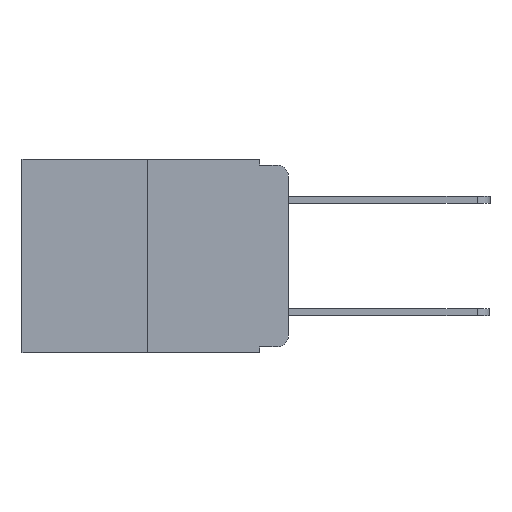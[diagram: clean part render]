
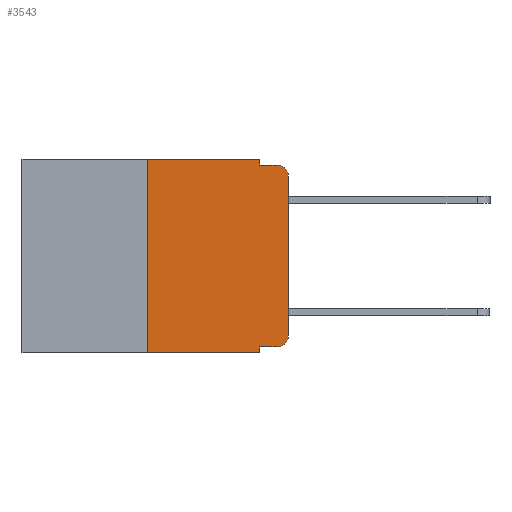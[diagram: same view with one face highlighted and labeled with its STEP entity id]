
A CAD part, left-side view. The second image highlights one B-rep face of the part: STEP entity #3543.
In plain terms, the highlighted planar face has unit normal (-1, 0, 0).
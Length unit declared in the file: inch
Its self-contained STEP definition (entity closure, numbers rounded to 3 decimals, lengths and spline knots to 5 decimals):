
#11 = VECTOR ( 'NONE', #3210, 39.37008 ) ;
#379 = VERTEX_POINT ( 'NONE', #9284 ) ;
#390 = DIRECTION ( 'NONE',  ( 0., -1., 0. ) ) ;
#411 = VERTEX_POINT ( 'NONE', #7543 ) ;
#413 = VECTOR ( 'NONE', #2440, 39.37008 ) ;
#439 = CIRCLE ( 'NONE', #7795, 0.02 ) ;
#510 = CARTESIAN_POINT ( 'NONE',  ( 0., 0.25, -0.343 ) ) ;
#577 = EDGE_CURVE ( 'NONE', #2965, #7936, #9200, .T. ) ;
#723 = CIRCLE ( 'NONE', #7772, 0.02 ) ;
#791 = VERTEX_POINT ( 'NONE', #5559 ) ;
#1036 = ORIENTED_EDGE ( 'NONE', *, *, #3986, .F. ) ;
#1056 = EDGE_CURVE ( 'NONE', #1644, #791, #4776, .T. ) ;
#1252 = VECTOR ( 'NONE', #7846, 39.37008 ) ;
#1349 = EDGE_CURVE ( 'NONE', #4883, #411, #8295, .T. ) ;
#1644 = VERTEX_POINT ( 'NONE', #3307 ) ;
#1993 = CARTESIAN_POINT ( 'NONE',  ( 0., 0.25, 0. ) ) ;
#2428 = CARTESIAN_POINT ( 'NONE',  ( 0., 0.051, -0.343 ) ) ;
#2440 = DIRECTION ( 'NONE',  ( 0., 0., 1. ) ) ;
#2455 = CARTESIAN_POINT ( 'NONE',  ( 0., 0.051, -0.333 ) ) ;
#2567 = DIRECTION ( 'NONE',  ( 0., -1., 0. ) ) ;
#2569 = AXIS2_PLACEMENT_3D ( 'NONE', #3844, #3490, #7368 ) ;
#2606 = CARTESIAN_POINT ( 'NONE',  ( 0., 0.02, -0.313 ) ) ;
#2618 = EDGE_CURVE ( 'NONE', #5900, #379, #8973, .T. ) ;
#2965 = VERTEX_POINT ( 'NONE', #510 ) ;
#2980 = CARTESIAN_POINT ( 'NONE',  ( 0., 0., -0.313 ) ) ;
#3188 = EDGE_CURVE ( 'NONE', #3818, #5900, #5981, .T. ) ;
#3210 = DIRECTION ( 'NONE',  ( 0., 0., -1. ) ) ;
#3298 = CARTESIAN_POINT ( 'NONE',  ( 0., 0.25, 0. ) ) ;
#3307 = CARTESIAN_POINT ( 'NONE',  ( 0., 0.051, -0.333 ) ) ;
#3315 = VECTOR ( 'NONE', #7057, 39.37008 ) ;
#3391 = CARTESIAN_POINT ( 'NONE',  ( 0., 0.051, 0. ) ) ;
#3412 = DIRECTION ( 'NONE',  ( 0., 0., -1. ) ) ;
#3490 = DIRECTION ( 'NONE',  ( 1., 0., 0. ) ) ;
#3543 = ADVANCED_FACE ( 'NONE', ( #7759 ), #7312, .F. ) ;
#3812 = CARTESIAN_POINT ( 'NONE',  ( 0., 0.051, -0.01 ) ) ;
#3818 = VERTEX_POINT ( 'NONE', #5576 ) ;
#3844 = CARTESIAN_POINT ( 'NONE',  ( 0., 0.473, 0. ) ) ;
#3855 = DIRECTION ( 'NONE',  ( -1., 0., 0. ) ) ;
#3986 = EDGE_CURVE ( 'NONE', #2965, #8779, #4206, .T. ) ;
#4033 = ORIENTED_EDGE ( 'NONE', *, *, #1056, .T. ) ;
#4055 = EDGE_CURVE ( 'NONE', #8779, #3818, #8850, .T. ) ;
#4173 = EDGE_LOOP ( 'NONE', ( #8802, #6750, #8694, #5788, #8195, #1036, #9188, #9390, #4033, #4270 ) ) ;
#4206 = LINE ( 'NONE', #3298, #6390 ) ;
#4270 = ORIENTED_EDGE ( 'NONE', *, *, #8054, .T. ) ;
#4776 = LINE ( 'NONE', #2455, #8397 ) ;
#4883 = VERTEX_POINT ( 'NONE', #2980 ) ;
#5002 = VECTOR ( 'NONE', #8585, 39.37008 ) ;
#5559 = CARTESIAN_POINT ( 'NONE',  ( 0., 0.02, -0.333 ) ) ;
#5576 = CARTESIAN_POINT ( 'NONE',  ( 0., 0.051, 0. ) ) ;
#5590 = LINE ( 'NONE', #3391, #3315 ) ;
#5788 = ORIENTED_EDGE ( 'NONE', *, *, #3188, .F. ) ;
#5900 = VERTEX_POINT ( 'NONE', #3812 ) ;
#5915 = CARTESIAN_POINT ( 'NONE',  ( 0., 0.051, 0. ) ) ;
#5947 = CARTESIAN_POINT ( 'NONE',  ( 0., 0.473, 0. ) ) ;
#5981 = LINE ( 'NONE', #5915, #11 ) ;
#6390 = VECTOR ( 'NONE', #7653, 39.37008 ) ;
#6428 = CARTESIAN_POINT ( 'NONE',  ( 0., 0., 0. ) ) ;
#6451 = EDGE_CURVE ( 'NONE', #411, #379, #439, .T. ) ;
#6750 = ORIENTED_EDGE ( 'NONE', *, *, #6451, .T. ) ;
#6755 = DIRECTION ( 'NONE',  ( 0., 0., -1. ) ) ;
#7057 = DIRECTION ( 'NONE',  ( 0., 0., -1. ) ) ;
#7105 = VECTOR ( 'NONE', #390, 39.37008 ) ;
#7312 = PLANE ( 'NONE',  #2569 ) ;
#7368 = DIRECTION ( 'NONE',  ( 0., 0., -1. ) ) ;
#7543 = CARTESIAN_POINT ( 'NONE',  ( 0., 0., -0.03 ) ) ;
#7653 = DIRECTION ( 'NONE',  ( 0., 0., 1. ) ) ;
#7733 = DIRECTION ( 'NONE',  ( -1., 0., 0. ) ) ;
#7759 = FACE_OUTER_BOUND ( 'NONE', #4173, .T. ) ;
#7772 = AXIS2_PLACEMENT_3D ( 'NONE', #2606, #7733, #3412 ) ;
#7795 = AXIS2_PLACEMENT_3D ( 'NONE', #8081, #3855, #6755 ) ;
#7846 = DIRECTION ( 'NONE',  ( 0., -1., 0. ) ) ;
#7936 = VERTEX_POINT ( 'NONE', #2428 ) ;
#7969 = CARTESIAN_POINT ( 'NONE',  ( 0., 0.051, -0.01 ) ) ;
#8054 = EDGE_CURVE ( 'NONE', #791, #4883, #723, .T. ) ;
#8081 = CARTESIAN_POINT ( 'NONE',  ( 0., 0.02, -0.03 ) ) ;
#8195 = ORIENTED_EDGE ( 'NONE', *, *, #4055, .F. ) ;
#8295 = LINE ( 'NONE', #6428, #413 ) ;
#8397 = VECTOR ( 'NONE', #2567, 39.37008 ) ;
#8578 = CARTESIAN_POINT ( 'NONE',  ( 0., 0.473, -0.343 ) ) ;
#8585 = DIRECTION ( 'NONE',  ( 0., -1., 0. ) ) ;
#8694 = ORIENTED_EDGE ( 'NONE', *, *, #2618, .F. ) ;
#8779 = VERTEX_POINT ( 'NONE', #1993 ) ;
#8802 = ORIENTED_EDGE ( 'NONE', *, *, #1349, .T. ) ;
#8850 = LINE ( 'NONE', #5947, #7105 ) ;
#8973 = LINE ( 'NONE', #7969, #1252 ) ;
#9188 = ORIENTED_EDGE ( 'NONE', *, *, #577, .T. ) ;
#9200 = LINE ( 'NONE', #8578, #5002 ) ;
#9281 = EDGE_CURVE ( 'NONE', #1644, #7936, #5590, .T. ) ;
#9284 = CARTESIAN_POINT ( 'NONE',  ( 0., 0.02, -0.01 ) ) ;
#9390 = ORIENTED_EDGE ( 'NONE', *, *, #9281, .F. ) ;
